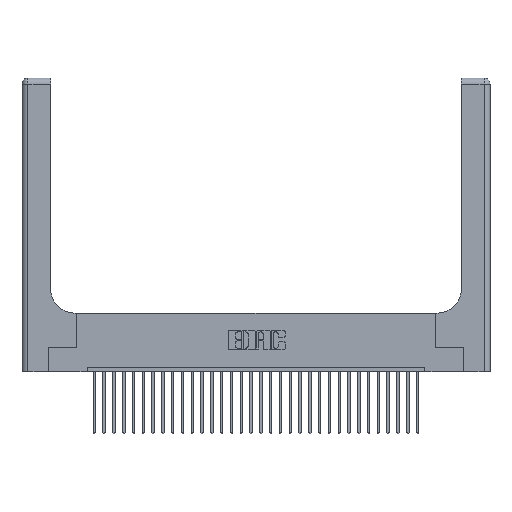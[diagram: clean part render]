
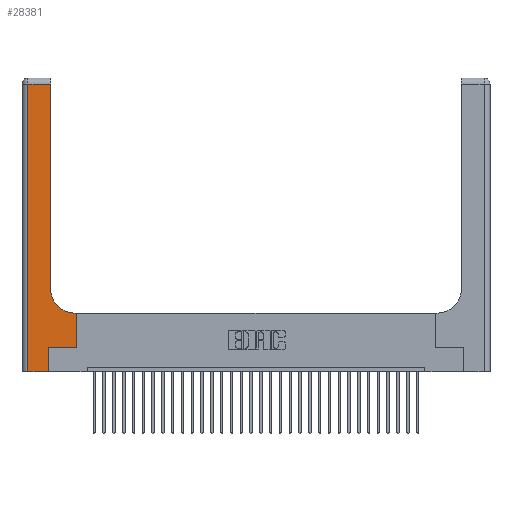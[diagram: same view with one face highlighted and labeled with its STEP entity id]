
A CAD part, top view. The second image highlights one B-rep face of the part: STEP entity #28381.
In plain terms, the highlighted planar face has unit normal (0, 0, 1).
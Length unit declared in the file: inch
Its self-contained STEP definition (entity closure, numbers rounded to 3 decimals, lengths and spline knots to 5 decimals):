
#604 = DIRECTION ( 'NONE',  ( 0., -1., 0. ) ) ;
#823 = CARTESIAN_POINT ( 'NONE',  ( 0.06, 3., 0.37 ) ) ;
#839 = DIRECTION ( 'NONE',  ( 0., 1., 0. ) ) ;
#1450 = CIRCLE ( 'NONE', #17339, 0.25 ) ;
#2712 = VERTEX_POINT ( 'NONE', #29404 ) ;
#2855 = VECTOR ( 'NONE', #26242, 39.37008 ) ;
#3308 = EDGE_CURVE ( 'NONE', #4203, #2712, #27595, .T. ) ;
#3422 = LINE ( 'NONE', #4743, #28810 ) ;
#3711 = ORIENTED_EDGE ( 'NONE', *, *, #8258, .T. ) ;
#4000 = CARTESIAN_POINT ( 'NONE',  ( 0.06, 0., 0.37 ) ) ;
#4203 = VERTEX_POINT ( 'NONE', #27008 ) ;
#4743 = CARTESIAN_POINT ( 'NONE',  ( 0.2915, 0.6, 0.37 ) ) ;
#4844 = EDGE_CURVE ( 'NONE', #5247, #17715, #12121, .T. ) ;
#5247 = VERTEX_POINT ( 'NONE', #9436 ) ;
#5565 = VECTOR ( 'NONE', #604, 39.37008 ) ;
#5623 = VERTEX_POINT ( 'NONE', #29854 ) ;
#5689 = CARTESIAN_POINT ( 'NONE',  ( 0.5585, 0.25, 0.37 ) ) ;
#6944 = DIRECTION ( 'NONE',  ( 0., 1., 0. ) ) ;
#7993 = VECTOR ( 'NONE', #22270, 39.37008 ) ;
#8206 = VECTOR ( 'NONE', #29999, 39.37008 ) ;
#8258 = EDGE_CURVE ( 'NONE', #5623, #20116, #3422, .T. ) ;
#8344 = PLANE ( 'NONE',  #18296 ) ;
#8607 = ORIENTED_EDGE ( 'NONE', *, *, #24505, .T. ) ;
#9436 = CARTESIAN_POINT ( 'NONE',  ( 0.06, 2.94, 0.37 ) ) ;
#9478 = CARTESIAN_POINT ( 'NONE',  ( 0.5415, 0.85, 0.37 ) ) ;
#9936 = CARTESIAN_POINT ( 'NONE',  ( 0.269, 0.25, 0.37 ) ) ;
#10188 = ORIENTED_EDGE ( 'NONE', *, *, #19455, .T. ) ;
#10557 = FACE_OUTER_BOUND ( 'NONE', #17936, .T. ) ;
#10567 = LINE ( 'NONE', #26807, #11732 ) ;
#11732 = VECTOR ( 'NONE', #12837, 39.37008 ) ;
#12060 = DIRECTION ( 'NONE',  ( -1., 0., 0. ) ) ;
#12121 = LINE ( 'NONE', #823, #5565 ) ;
#12594 = LINE ( 'NONE', #26475, #21039 ) ;
#12837 = DIRECTION ( 'NONE',  ( -1., 0., 0. ) ) ;
#13379 = VERTEX_POINT ( 'NONE', #5689 ) ;
#13866 = ORIENTED_EDGE ( 'NONE', *, *, #28823, .T. ) ;
#14794 = LINE ( 'NONE', #27646, #8206 ) ;
#14855 = EDGE_CURVE ( 'NONE', #2712, #5247, #10567, .T. ) ;
#15313 = CARTESIAN_POINT ( 'NONE',  ( 0.269, 0., 0.37 ) ) ;
#16550 = ORIENTED_EDGE ( 'NONE', *, *, #14855, .T. ) ;
#17248 = VERTEX_POINT ( 'NONE', #15313 ) ;
#17339 = AXIS2_PLACEMENT_3D ( 'NONE', #9478, #26664, #21858 ) ;
#17360 = CARTESIAN_POINT ( 'NONE',  ( 0.2915, 3., 0.37 ) ) ;
#17513 = LINE ( 'NONE', #28598, #2855 ) ;
#17715 = VERTEX_POINT ( 'NONE', #4000 ) ;
#17936 = EDGE_LOOP ( 'NONE', ( #29164, #16550, #26414, #13866, #8607, #23525, #29094, #3711, #10188 ) ) ;
#18296 = AXIS2_PLACEMENT_3D ( 'NONE', #20821, #20631, #25536 ) ;
#18893 = VERTEX_POINT ( 'NONE', #9936 ) ;
#19455 = EDGE_CURVE ( 'NONE', #20116, #4203, #1450, .T. ) ;
#19637 = LINE ( 'NONE', #27605, #22321 ) ;
#20116 = VERTEX_POINT ( 'NONE', #29175 ) ;
#20631 = DIRECTION ( 'NONE',  ( 0., 0., -1. ) ) ;
#20821 = CARTESIAN_POINT ( 'NONE',  ( 0., 3., 0.37 ) ) ;
#21039 = VECTOR ( 'NONE', #6944, 39.37008 ) ;
#21858 = DIRECTION ( 'NONE',  ( 1., 0., 0. ) ) ;
#22270 = DIRECTION ( 'NONE',  ( 0., 1., 0. ) ) ;
#22321 = VECTOR ( 'NONE', #839, 39.37008 ) ;
#23525 = ORIENTED_EDGE ( 'NONE', *, *, #25846, .T. ) ;
#24505 = EDGE_CURVE ( 'NONE', #17248, #18893, #12594, .T. ) ;
#25536 = DIRECTION ( 'NONE',  ( -1., 0., 0. ) ) ;
#25846 = EDGE_CURVE ( 'NONE', #18893, #13379, #17513, .T. ) ;
#26242 = DIRECTION ( 'NONE',  ( 1., 0., 0. ) ) ;
#26414 = ORIENTED_EDGE ( 'NONE', *, *, #4844, .T. ) ;
#26475 = CARTESIAN_POINT ( 'NONE',  ( 0.269, 0., 0.37 ) ) ;
#26664 = DIRECTION ( 'NONE',  ( 0., 0., -1. ) ) ;
#26807 = CARTESIAN_POINT ( 'NONE',  ( 0., 2.94, 0.37 ) ) ;
#27008 = CARTESIAN_POINT ( 'NONE',  ( 0.2915, 0.85, 0.37 ) ) ;
#27595 = LINE ( 'NONE', #17360, #7993 ) ;
#27605 = CARTESIAN_POINT ( 'NONE',  ( 0.5585, 0.25, 0.37 ) ) ;
#27646 = CARTESIAN_POINT ( 'NONE',  ( 0., 0., 0.37 ) ) ;
#28381 = ADVANCED_FACE ( 'NONE', ( #10557 ), #8344, .F. ) ;
#28598 = CARTESIAN_POINT ( 'NONE',  ( 0.269, 0.25, 0.37 ) ) ;
#28810 = VECTOR ( 'NONE', #12060, 39.37008 ) ;
#28823 = EDGE_CURVE ( 'NONE', #17715, #17248, #14794, .T. ) ;
#29094 = ORIENTED_EDGE ( 'NONE', *, *, #31778, .T. ) ;
#29164 = ORIENTED_EDGE ( 'NONE', *, *, #3308, .T. ) ;
#29175 = CARTESIAN_POINT ( 'NONE',  ( 0.5415, 0.6, 0.37 ) ) ;
#29404 = CARTESIAN_POINT ( 'NONE',  ( 0.2915, 2.94, 0.37 ) ) ;
#29854 = CARTESIAN_POINT ( 'NONE',  ( 0.5585, 0.6, 0.37 ) ) ;
#29999 = DIRECTION ( 'NONE',  ( 1., 0., 0. ) ) ;
#31778 = EDGE_CURVE ( 'NONE', #13379, #5623, #19637, .T. ) ;
